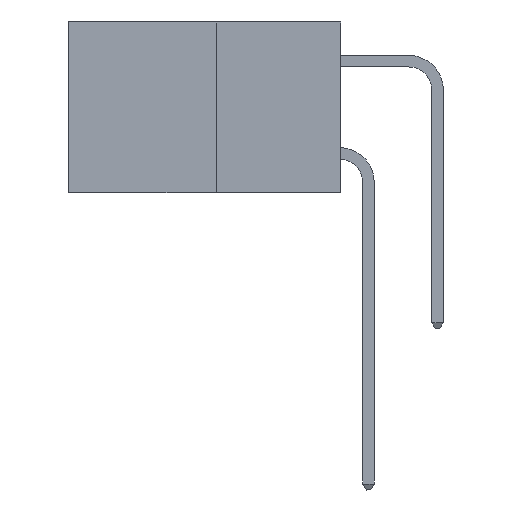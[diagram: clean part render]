
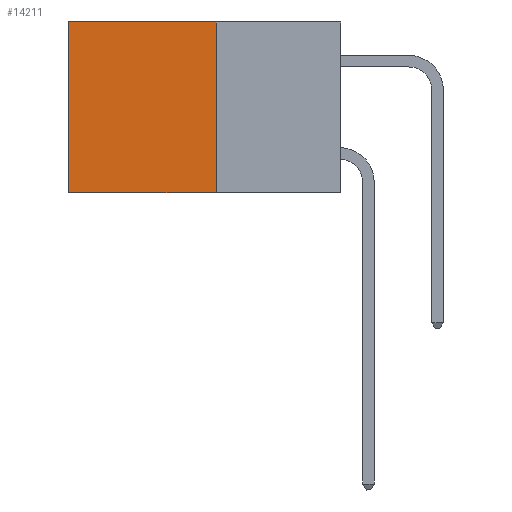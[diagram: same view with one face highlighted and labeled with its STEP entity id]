
A CAD part, left-side view. The second image highlights one B-rep face of the part: STEP entity #14211.
In plain terms, the highlighted planar face has unit normal (-1, 0, 0).
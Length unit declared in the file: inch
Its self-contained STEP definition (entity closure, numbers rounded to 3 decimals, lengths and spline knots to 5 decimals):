
#79 = ORIENTED_EDGE ( 'NONE', *, *, #8049, .F. ) ;
#327 = DIRECTION ( 'NONE',  ( 0., 0., -1. ) ) ;
#491 = AXIS2_PLACEMENT_3D ( 'NONE', #12189, #16301, #7906 ) ;
#828 = ORIENTED_EDGE ( 'NONE', *, *, #3261, .F. ) ;
#994 = VECTOR ( 'NONE', #14091, 39.37008 ) ;
#1175 = CARTESIAN_POINT ( 'NONE',  ( 0.277, 0.59, 0. ) ) ;
#1295 = ORIENTED_EDGE ( 'NONE', *, *, #9091, .T. ) ;
#1711 = LINE ( 'NONE', #10565, #12960 ) ;
#2874 = CARTESIAN_POINT ( 'NONE',  ( 0.277, 0.27, -0.37 ) ) ;
#3261 = EDGE_CURVE ( 'NONE', #4643, #11725, #13945, .T. ) ;
#4128 = CARTESIAN_POINT ( 'NONE',  ( 0.277, 0.59, -0.37 ) ) ;
#4351 = VERTEX_POINT ( 'NONE', #4128 ) ;
#4643 = VERTEX_POINT ( 'NONE', #11845 ) ;
#5687 = EDGE_LOOP ( 'NONE', ( #18347, #79, #828, #1295 ) ) ;
#7852 = EDGE_CURVE ( 'NONE', #15125, #4351, #12766, .T. ) ;
#7906 = DIRECTION ( 'NONE',  ( 0., 0., -1. ) ) ;
#8049 = EDGE_CURVE ( 'NONE', #11725, #4351, #1711, .T. ) ;
#8188 = CARTESIAN_POINT ( 'NONE',  ( 0.277, 0.27, -0.37 ) ) ;
#8225 = VECTOR ( 'NONE', #11698, 39.37008 ) ;
#9091 = EDGE_CURVE ( 'NONE', #4643, #15125, #16118, .T. ) ;
#10537 = DIRECTION ( 'NONE',  ( 0., 1., 0. ) ) ;
#10565 = CARTESIAN_POINT ( 'NONE',  ( 0.277, 0.27, -0.37 ) ) ;
#10873 = FACE_OUTER_BOUND ( 'NONE', #5687, .T. ) ;
#11698 = DIRECTION ( 'NONE',  ( 0., 1., 0. ) ) ;
#11725 = VERTEX_POINT ( 'NONE', #2874 ) ;
#11845 = CARTESIAN_POINT ( 'NONE',  ( 0.277, 0.27, 0. ) ) ;
#12189 = CARTESIAN_POINT ( 'NONE',  ( 0.277, 0.27, -0.37 ) ) ;
#12766 = LINE ( 'NONE', #14124, #994 ) ;
#12960 = VECTOR ( 'NONE', #10537, 39.37008 ) ;
#13024 = CARTESIAN_POINT ( 'NONE',  ( 0.277, 0.27, 0. ) ) ;
#13945 = LINE ( 'NONE', #8188, #17517 ) ;
#14091 = DIRECTION ( 'NONE',  ( 0., 0., -1. ) ) ;
#14124 = CARTESIAN_POINT ( 'NONE',  ( 0.277, 0.59, -0.37 ) ) ;
#14211 = ADVANCED_FACE ( 'NONE', ( #10873 ), #16237, .F. ) ;
#15125 = VERTEX_POINT ( 'NONE', #1175 ) ;
#16118 = LINE ( 'NONE', #13024, #8225 ) ;
#16237 = PLANE ( 'NONE',  #491 ) ;
#16301 = DIRECTION ( 'NONE',  ( 1., 0., 0. ) ) ;
#17517 = VECTOR ( 'NONE', #327, 39.37008 ) ;
#18347 = ORIENTED_EDGE ( 'NONE', *, *, #7852, .T. ) ;
